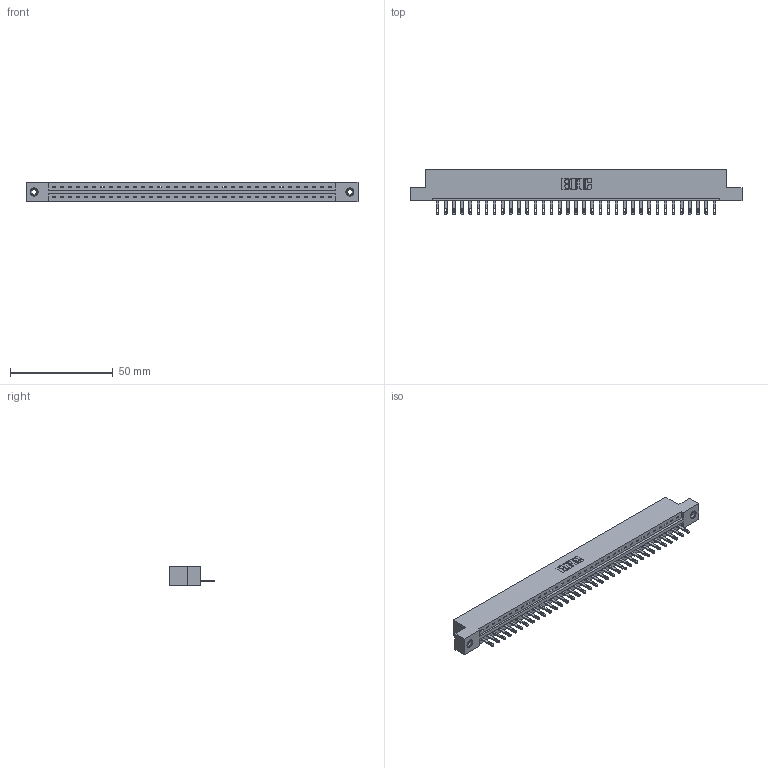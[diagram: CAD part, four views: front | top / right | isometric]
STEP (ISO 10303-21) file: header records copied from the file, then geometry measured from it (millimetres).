
FILE_DESCRIPTION (( 'STEP AP203' ), '1' );
FILE_NAME ('887-035-500-108.STEP', '2020-09-20T21:58:16', ( '' ), ( '' ), 'SwSTEP 2.0', 'SolidWorks 2020', '' );
FILE_SCHEMA (( 'CONFIG_CONTROL_DESIGN' ));
Length unit declared in the file: inch
Products named in the file (4): 837 Part_Flush Mounting Lugs - 0.156 Dia-TI; 345-250-001_345-250-003-102; 345-292-001_345-293-100; 887-035-500-108
Assembly tree (38 placements, depth 2):
  887-035-500-108
    837 Part_Flush Mounting Lugs - 0.156 Dia-TI
    345-292-001_345-293-100  x35
    345-250-001_345-250-003-102  x2
Bounding box: 161.7 x 21.85 x 9.4 mm (x, y, z)
Volume: 16733.2 mm3; surface area: 17363.8 mm2
Topology: 38 solids, 38 shells, 2204 faces, 6747 edges, 4490 vertices
Faces by surface type: plane 1502, cylinder 686, cone 12, torus 4
Entity records: 28038 total; most frequent: CARTESIAN_POINT 4862, ORIENTED_EDGE 4826, DIRECTION 4141, EDGE_CURVE 2413, VECTOR 2261, LINE 2261, VERTEX_POINT 1604, AXIS2_PLACEMENT_3D 940
